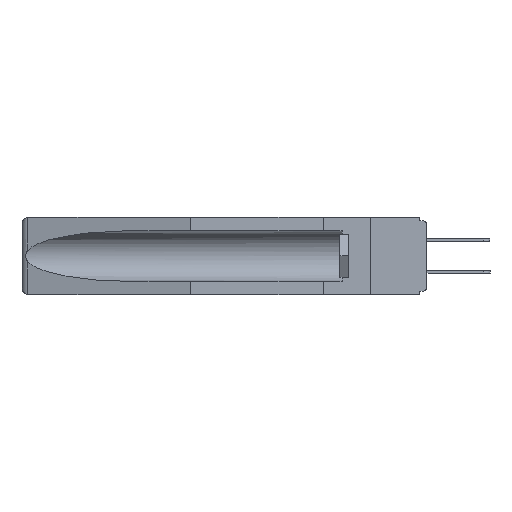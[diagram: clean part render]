
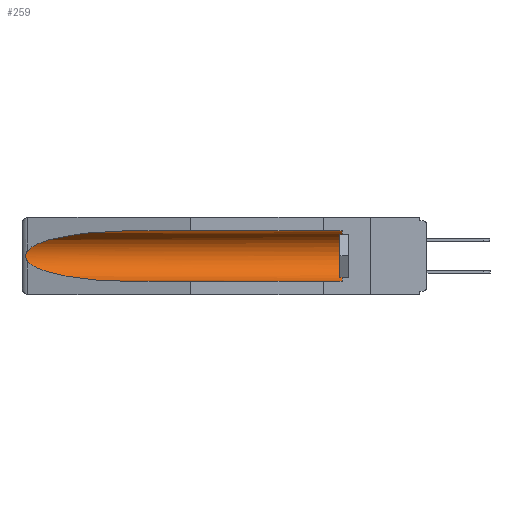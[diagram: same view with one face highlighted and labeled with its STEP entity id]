
A CAD part, left-side view. The second image highlights one B-rep face of the part: STEP entity #259.
In plain terms, the highlighted cylindrical face has radius 2.857 mm (diameter 5.715 mm), a partial arc.
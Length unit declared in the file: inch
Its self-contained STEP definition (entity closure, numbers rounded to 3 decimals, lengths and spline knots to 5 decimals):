
#97 = DIRECTION ( 'NONE',  ( 0., 1., 0. ) ) ;
#213 = CARTESIAN_POINT ( 'NONE',  ( 0.26537, 1.52718, -0.19328 ) ) ;
#259 = ADVANCED_FACE ( 'NONE', ( #19644 ), #16496, .F. ) ;
#767 = EDGE_LOOP ( 'NONE', ( #15174, #3826, #15827, #10976, #8682, #4326 ) ) ;
#991 = CARTESIAN_POINT ( 'NONE',  ( 0.26597, 1.52961, -0.15275 ) ) ;
#1392 = DIRECTION ( 'NONE',  ( 0., -1., 0. ) ) ;
#2027 = CARTESIAN_POINT ( 'NONE',  ( 0.155, -0.30754, -0.059 ) ) ;
#2580 = CARTESIAN_POINT ( 'NONE',  ( 0.26654, 1.53092, -0.15636 ) ) ;
#2899 = CARTESIAN_POINT ( 'NONE',  ( 0.25451, 1.48313, -0.09465 ) ) ;
#3601 = DIRECTION ( 'NONE',  ( 0., 1., 0. ) ) ;
#3826 = ORIENTED_EDGE ( 'NONE', *, *, #5507, .T. ) ;
#4326 = ORIENTED_EDGE ( 'NONE', *, *, #11477, .T. ) ;
#4775 = CARTESIAN_POINT ( 'NONE',  ( 0.25451, 1.48313, -0.24835 ) ) ;
#5090 = EDGE_CURVE ( 'NONE', #18477, #12342, #11423, .T. ) ;
#5287 = CARTESIAN_POINT ( 'NONE',  ( 0.26537, 1.52718, -0.14972 ) ) ;
#5507 = EDGE_CURVE ( 'NONE', #8418, #17479, #9280, .T. ) ;
#5572 = EDGE_CURVE ( 'NONE', #15683, #8418, #17071, .T. ) ;
#5687 = CARTESIAN_POINT ( 'NONE',  ( 0.26537, 1.52718, -0.19328 ) ) ;
#5813 = CARTESIAN_POINT ( 'NONE',  ( 0.2675, 1.53308, -0.16763 ) ) ;
#5832 = EDGE_CURVE ( 'NONE', #18477, #11793, #18881, .T. ) ;
#6133 = AXIS2_PLACEMENT_3D ( 'NONE', #9419, #97, #8038 ) ;
#6723 = EDGE_CURVE ( 'NONE', #17479, #12342, #18553, .T. ) ;
#7331 = VECTOR ( 'NONE', #3601, 39.37008 ) ;
#7439 = CARTESIAN_POINT ( 'NONE',  ( 0.21114, 1.30732, -0.059 ) ) ;
#8038 = DIRECTION ( 'NONE',  ( 0., 0., 1. ) ) ;
#8372 = DIRECTION ( 'NONE',  ( 0., 1., 0. ) ) ;
#8418 = VERTEX_POINT ( 'NONE', #5287 ) ;
#8682 = ORIENTED_EDGE ( 'NONE', *, *, #5832, .T. ) ;
#9280 = B_SPLINE_CURVE_WITH_KNOTS ( 'NONE', 3,
 ( #18017, #991, #2580, #18137, #5813, #11883, #10185, #11758, #14982, #5687 ),
 .UNSPECIFIED., .F., .F.,
 ( 4, 2, 2, 2, 4 ),
 ( 0., 0.00029, 0.00058, 0.00087, 0.00117 ),
 .UNSPECIFIED. ) ;
#9419 = CARTESIAN_POINT ( 'NONE',  ( 0.155, -0.30754, -0.1715 ) ) ;
#10185 = CARTESIAN_POINT ( 'NONE',  ( 0.2673, 1.53269, -0.17917 ) ) ;
#10403 = CARTESIAN_POINT ( 'NONE',  ( 0.155, 1.07973, -0.059 ) ) ;
#10976 = ORIENTED_EDGE ( 'NONE', *, *, #5090, .F. ) ;
#11082 = CARTESIAN_POINT ( 'NONE',  ( 0.21114, 1.30732, -0.284 ) ) ;
#11423 = LINE ( 'NONE', #14551, #17685 ) ;
#11477 = EDGE_CURVE ( 'NONE', #11793, #15683, #18484, .T. ) ;
#11758 = CARTESIAN_POINT ( 'NONE',  ( 0.26655, 1.53094, -0.18657 ) ) ;
#11793 = VERTEX_POINT ( 'NONE', #12614 ) ;
#11883 = CARTESIAN_POINT ( 'NONE',  ( 0.2675, 1.53308, -0.17534 ) ) ;
#12342 = VERTEX_POINT ( 'NONE', #14447 ) ;
#12515 = CARTESIAN_POINT ( 'NONE',  ( 0.155, 0.126, -0.284 ) ) ;
#12614 = CARTESIAN_POINT ( 'NONE',  ( 0.155, 0.126, -0.059 ) ) ;
#14447 = CARTESIAN_POINT ( 'NONE',  ( 0.155, 1.07973, -0.284 ) ) ;
#14551 = CARTESIAN_POINT ( 'NONE',  ( 0.155, -0.30754, -0.284 ) ) ;
#14982 = CARTESIAN_POINT ( 'NONE',  ( 0.26597, 1.5296, -0.19026 ) ) ;
#15174 = ORIENTED_EDGE ( 'NONE', *, *, #5572, .T. ) ;
#15185 = DIRECTION ( 'NONE',  ( 0., 0., 1. ) ) ;
#15501 = CARTESIAN_POINT ( 'NONE',  ( 0.26537, 1.52718, -0.14972 ) ) ;
#15582 = CARTESIAN_POINT ( 'NONE',  ( 0.26537, 1.52718, -0.19328 ) ) ;
#15616 = CARTESIAN_POINT ( 'NONE',  ( 0.155, 1.07973, -0.284 ) ) ;
#15683 = VERTEX_POINT ( 'NONE', #10403 ) ;
#15827 = ORIENTED_EDGE ( 'NONE', *, *, #6723, .T. ) ;
#16496 = CYLINDRICAL_SURFACE ( 'NONE', #6133, 0.1125 ) ;
#16723 = CARTESIAN_POINT ( 'NONE',  ( 0.155, 1.07973, -0.059 ) ) ;
#17071 =( BOUNDED_CURVE ( )  B_SPLINE_CURVE ( 3, ( #16723, #7439, #2899, #15501 ),
 .UNSPECIFIED., .F., .T. ) 
 B_SPLINE_CURVE_WITH_KNOTS ( ( 4, 4 ),
 ( 4.71239, 6.08839 ),
 .UNSPECIFIED. ) 
 CURVE ( )  GEOMETRIC_REPRESENTATION_ITEM ( )  RATIONAL_B_SPLINE_CURVE ( ( 1., 0.848, 0.848, 1. ) ) 
 REPRESENTATION_ITEM ( '' )  );
#17479 = VERTEX_POINT ( 'NONE', #15582 ) ;
#17685 = VECTOR ( 'NONE', #8372, 39.37008 ) ;
#18017 = CARTESIAN_POINT ( 'NONE',  ( 0.26537, 1.52718, -0.14972 ) ) ;
#18137 = CARTESIAN_POINT ( 'NONE',  ( 0.2673, 1.5327, -0.16383 ) ) ;
#18276 = CARTESIAN_POINT ( 'NONE',  ( 0.155, 0.126, -0.1715 ) ) ;
#18477 = VERTEX_POINT ( 'NONE', #12515 ) ;
#18484 = LINE ( 'NONE', #2027, #7331 ) ;
#18553 =( BOUNDED_CURVE ( )  B_SPLINE_CURVE ( 3, ( #213, #4775, #11082, #15616 ),
 .UNSPECIFIED., .F., .F. ) 
 B_SPLINE_CURVE_WITH_KNOTS ( ( 4, 4 ),
 ( 0.1948, 1.5708 ),
 .UNSPECIFIED. ) 
 CURVE ( )  GEOMETRIC_REPRESENTATION_ITEM ( )  RATIONAL_B_SPLINE_CURVE ( ( 1., 0.848, 0.848, 1. ) ) 
 REPRESENTATION_ITEM ( '' )  );
#18881 = CIRCLE ( 'NONE', #18908, 0.1125 ) ;
#18908 = AXIS2_PLACEMENT_3D ( 'NONE', #18276, #1392, #15185 ) ;
#19644 = FACE_OUTER_BOUND ( 'NONE', #767, .T. ) ;
